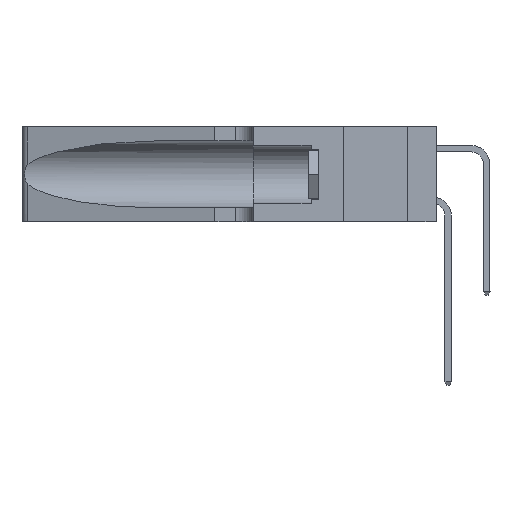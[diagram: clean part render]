
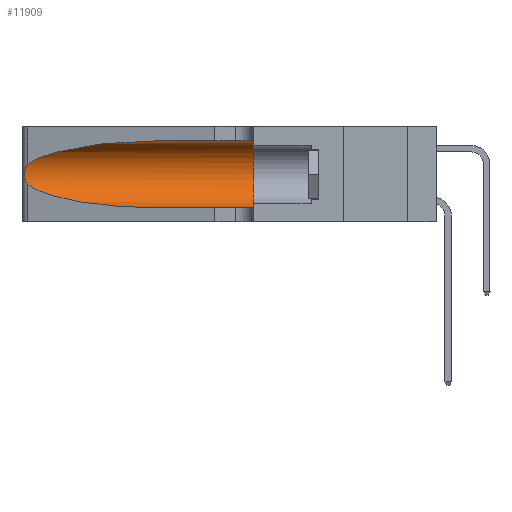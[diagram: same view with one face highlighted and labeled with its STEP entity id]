
A CAD part, left-side view. The second image highlights one B-rep face of the part: STEP entity #11909.
In plain terms, the highlighted cylindrical face has radius 3.308 mm (diameter 6.617 mm), a partial arc.
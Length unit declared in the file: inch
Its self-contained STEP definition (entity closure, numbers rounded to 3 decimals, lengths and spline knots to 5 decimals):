
#120 = EDGE_CURVE ( 'NONE', #11824, #12950, #2844, .T. ) ;
#532 = CARTESIAN_POINT ( 'NONE',  ( 0.1305, 0.72297, 0.05475 ) ) ;
#658 = DIRECTION ( 'NONE',  ( 0., 0., 1. ) ) ;
#1239 = EDGE_CURVE ( 'NONE', #23329, #13415, #8148, .T. ) ;
#1455 = CARTESIAN_POINT ( 'NONE',  ( 0.25854, 1.2359, 0.20912 ) ) ;
#2038 = CARTESIAN_POINT ( 'NONE',  ( 0.25487, 1.22718, 0.14631 ) ) ;
#2711 = CARTESIAN_POINT ( 'NONE',  ( 0.1305, 0.72297, 0.31525 ) ) ;
#2797 = CARTESIAN_POINT ( 'NONE',  ( 0.25487, 1.22718, 0.22369 ) ) ;
#2844 =( BOUNDED_CURVE ( )  B_SPLINE_CURVE ( 3, ( #2711, #8276, #10205, #2797 ),
 .UNSPECIFIED., .F., .T. ) 
 B_SPLINE_CURVE_WITH_KNOTS ( ( 4, 4 ),
 ( 1.5708, 2.84003 ),
 .UNSPECIFIED. ) 
 CURVE ( )  GEOMETRIC_REPRESENTATION_ITEM ( )  RATIONAL_B_SPLINE_CURVE ( ( 1., 0.87, 0.87, 1. ) ) 
 REPRESENTATION_ITEM ( '' )  );
#3079 = AXIS2_PLACEMENT_3D ( 'NONE', #22198, #11464, #20736 ) ;
#4186 = CARTESIAN_POINT ( 'NONE',  ( 0.25487, 1.22718, 0.14631 ) ) ;
#4196 = DIRECTION ( 'NONE',  ( 0., -1., 0. ) ) ;
#4402 = CARTESIAN_POINT ( 'NONE',  ( 0.1305, 0.35, 0.31525 ) ) ;
#4603 = CARTESIAN_POINT ( 'NONE',  ( 0.25639, 1.23184, 0.21858 ) ) ;
#4736 = VECTOR ( 'NONE', #4196, 39.37008 ) ;
#5269 = LINE ( 'NONE', #17988, #15669 ) ;
#5414 = CARTESIAN_POINT ( 'NONE',  ( 0.26075, 1.23896, 0.178 ) ) ;
#5805 = ORIENTED_EDGE ( 'NONE', *, *, #18888, .T. ) ;
#6139 = CARTESIAN_POINT ( 'NONE',  ( 0.25487, 1.22718, 0.22369 ) ) ;
#6568 = FACE_OUTER_BOUND ( 'NONE', #17435, .T. ) ;
#7194 = CARTESIAN_POINT ( 'NONE',  ( 0.25555, 1.22993, 0.14849 ) ) ;
#7260 = CARTESIAN_POINT ( 'NONE',  ( 0.25639, 1.23186, 0.15144 ) ) ;
#7605 = CARTESIAN_POINT ( 'NONE',  ( 0.18966, 0.96281, 0.05475 ) ) ;
#7754 = EDGE_CURVE ( 'NONE', #16833, #8992, #23693, .T. ) ;
#8148 =( BOUNDED_CURVE ( )  B_SPLINE_CURVE ( 3, ( #2038, #20585, #7605, #22453 ),
 .UNSPECIFIED., .F., .T. ) 
 B_SPLINE_CURVE_WITH_KNOTS ( ( 4, 4 ),
 ( 3.44316, 4.71239 ),
 .UNSPECIFIED. ) 
 CURVE ( )  GEOMETRIC_REPRESENTATION_ITEM ( )  RATIONAL_B_SPLINE_CURVE ( ( 1., 0.87, 0.87, 1. ) ) 
 REPRESENTATION_ITEM ( '' )  );
#8205 = LINE ( 'NONE', #15265, #4736 ) ;
#8276 = CARTESIAN_POINT ( 'NONE',  ( 0.18966, 0.96281, 0.31525 ) ) ;
#8992 = VERTEX_POINT ( 'NONE', #16542 ) ;
#9926 = B_SPLINE_CURVE_WITH_KNOTS ( 'NONE', 3,
 ( #6139, #22759, #4603, #17534, #1455, #22266, #14533, #5414, #16397, #12911, #16472, #7260, #7194, #14931 ),
 .UNSPECIFIED., .F., .F.,
 ( 4, 2, 2, 2, 2, 2, 4 ),
 ( 0., 0.00027, 0.00053, 0.00107, 0.0016, 0.00187, 0.00214 ),
 .UNSPECIFIED. ) ;
#10205 = CARTESIAN_POINT ( 'NONE',  ( 0.2373, 1.15595, 0.28018 ) ) ;
#10630 = CARTESIAN_POINT ( 'NONE',  ( 0.25487, 1.22718, 0.22369 ) ) ;
#11411 = ORIENTED_EDGE ( 'NONE', *, *, #20475, .F. ) ;
#11464 = DIRECTION ( 'NONE',  ( 0., -1., 0. ) ) ;
#11726 = ORIENTED_EDGE ( 'NONE', *, *, #1239, .T. ) ;
#11824 = VERTEX_POINT ( 'NONE', #12615 ) ;
#11909 = ADVANCED_FACE ( 'NONE', ( #6568 ), #22714, .F. ) ;
#12615 = CARTESIAN_POINT ( 'NONE',  ( 0.1305, 0.72297, 0.31525 ) ) ;
#12911 = CARTESIAN_POINT ( 'NONE',  ( 0.25856, 1.23593, 0.16098 ) ) ;
#12950 = VERTEX_POINT ( 'NONE', #10630 ) ;
#13415 = VERTEX_POINT ( 'NONE', #532 ) ;
#14262 = ORIENTED_EDGE ( 'NONE', *, *, #20812, .T. ) ;
#14533 = CARTESIAN_POINT ( 'NONE',  ( 0.26075, 1.23896, 0.19203 ) ) ;
#14931 = CARTESIAN_POINT ( 'NONE',  ( 0.25487, 1.22718, 0.14631 ) ) ;
#15265 = CARTESIAN_POINT ( 'NONE',  ( 0.1305, 1.61858, 0.05475 ) ) ;
#15669 = VECTOR ( 'NONE', #21614, 39.37008 ) ;
#15846 = ORIENTED_EDGE ( 'NONE', *, *, #120, .T. ) ;
#16397 = CARTESIAN_POINT ( 'NONE',  ( 0.26017, 1.23833, 0.17102 ) ) ;
#16472 = CARTESIAN_POINT ( 'NONE',  ( 0.25789, 1.23486, 0.15765 ) ) ;
#16542 = CARTESIAN_POINT ( 'NONE',  ( 0.1305, 0.35, 0.05475 ) ) ;
#16833 = VERTEX_POINT ( 'NONE', #4402 ) ;
#17156 = CARTESIAN_POINT ( 'NONE',  ( 0.1305, 0.35, 0.185 ) ) ;
#17406 = DIRECTION ( 'NONE',  ( 0., 1., 0. ) ) ;
#17435 = EDGE_LOOP ( 'NONE', ( #15846, #14262, #11726, #5805, #19573, #11411 ) ) ;
#17534 = CARTESIAN_POINT ( 'NONE',  ( 0.25787, 1.23484, 0.2124 ) ) ;
#17988 = CARTESIAN_POINT ( 'NONE',  ( 0.1305, 1.61858, 0.31525 ) ) ;
#18888 = EDGE_CURVE ( 'NONE', #13415, #8992, #8205, .T. ) ;
#19573 = ORIENTED_EDGE ( 'NONE', *, *, #7754, .F. ) ;
#20475 = EDGE_CURVE ( 'NONE', #11824, #16833, #5269, .T. ) ;
#20585 = CARTESIAN_POINT ( 'NONE',  ( 0.2373, 1.15595, 0.08982 ) ) ;
#20736 = DIRECTION ( 'NONE',  ( 0., 0., -1. ) ) ;
#20812 = EDGE_CURVE ( 'NONE', #12950, #23329, #9926, .T. ) ;
#21614 = DIRECTION ( 'NONE',  ( 0., -1., 0. ) ) ;
#22198 = CARTESIAN_POINT ( 'NONE',  ( 0.1305, 1.61858, 0.185 ) ) ;
#22266 = CARTESIAN_POINT ( 'NONE',  ( 0.26018, 1.23835, 0.19895 ) ) ;
#22453 = CARTESIAN_POINT ( 'NONE',  ( 0.1305, 0.72297, 0.05475 ) ) ;
#22714 = CYLINDRICAL_SURFACE ( 'NONE', #3079, 0.13025 ) ;
#22759 = CARTESIAN_POINT ( 'NONE',  ( 0.25555, 1.22994, 0.2215 ) ) ;
#22806 = AXIS2_PLACEMENT_3D ( 'NONE', #17156, #17406, #658 ) ;
#23329 = VERTEX_POINT ( 'NONE', #4186 ) ;
#23693 = CIRCLE ( 'NONE', #22806, 0.13025 ) ;
